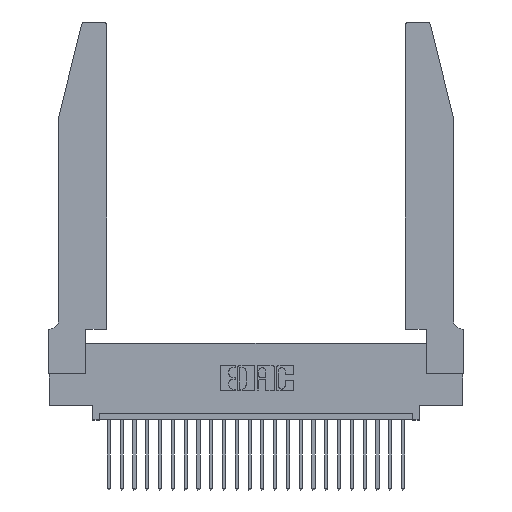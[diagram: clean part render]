
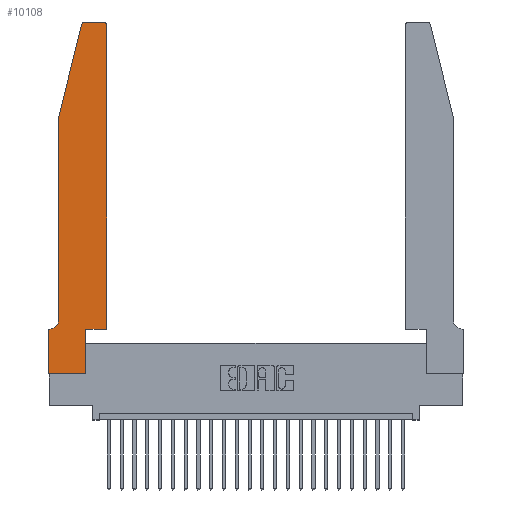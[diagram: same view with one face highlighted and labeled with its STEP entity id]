
A CAD part, top view. The second image highlights one B-rep face of the part: STEP entity #10108.
In plain terms, the highlighted planar face has unit normal (0, 0, 1).
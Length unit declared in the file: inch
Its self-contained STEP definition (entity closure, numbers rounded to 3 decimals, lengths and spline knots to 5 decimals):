
#411 = DIRECTION ( 'NONE',  ( 0., 0., 1. ) ) ;
#413 = LINE ( 'NONE', #1307, #14219 ) ;
#421 = CARTESIAN_POINT ( 'NONE',  ( 0.2605, 2.75, 0.37 ) ) ;
#437 = DIRECTION ( 'NONE',  ( 0., 1., 0. ) ) ;
#847 = VECTOR ( 'NONE', #10020, 39.37008 ) ;
#921 = EDGE_CURVE ( 'NONE', #11920, #24550, #14536, .T. ) ;
#956 = CARTESIAN_POINT ( 'NONE',  ( 0.4505, 0.35, 0.37 ) ) ;
#1104 = EDGE_CURVE ( 'NONE', #2616, #14932, #413, .T. ) ;
#1137 = VERTEX_POINT ( 'NONE', #4979 ) ;
#1307 = CARTESIAN_POINT ( 'NONE',  ( 0., 0., 0.37 ) ) ;
#1607 = EDGE_CURVE ( 'NONE', #24550, #12970, #20938, .T. ) ;
#1717 = CARTESIAN_POINT ( 'NONE',  ( 0.284, 2.75, 0.37 ) ) ;
#2001 = CIRCLE ( 'NONE', #3855, 0.07 ) ;
#2033 = DIRECTION ( 'NONE',  ( 0., 0., 1. ) ) ;
#2428 = CARTESIAN_POINT ( 'NONE',  ( 0.0755, 2., 0.37 ) ) ;
#2616 = VERTEX_POINT ( 'NONE', #12518 ) ;
#2748 = ORIENTED_EDGE ( 'NONE', *, *, #10962, .T. ) ;
#2857 = VECTOR ( 'NONE', #20580, 39.37008 ) ;
#3002 = FACE_OUTER_BOUND ( 'NONE', #3259, .T. ) ;
#3259 = EDGE_LOOP ( 'NONE', ( #16707, #22933, #7563, #19313, #4083, #14543, #13336, #22594, #2748, #11919, #10483, #11389 ) ) ;
#3855 = AXIS2_PLACEMENT_3D ( 'NONE', #16775, #8666, #4684 ) ;
#3896 = CIRCLE ( 'NONE', #11176, 0.03 ) ;
#3899 = CIRCLE ( 'NONE', #13970, 0.03 ) ;
#4083 = ORIENTED_EDGE ( 'NONE', *, *, #6516, .T. ) ;
#4098 = CARTESIAN_POINT ( 'NONE',  ( 0.4505, 0.35, 0.37 ) ) ;
#4505 = EDGE_CURVE ( 'NONE', #8027, #13186, #14383, .T. ) ;
#4684 = DIRECTION ( 'NONE',  ( -1., 0., 0. ) ) ;
#4979 = CARTESIAN_POINT ( 'NONE',  ( 0., 0.35, 0.37 ) ) ;
#5818 = CARTESIAN_POINT ( 'NONE',  ( 0.284, 2.72, 0.37 ) ) ;
#6023 = CARTESIAN_POINT ( 'NONE',  ( 0.0755, 0.42, 0.37 ) ) ;
#6516 = EDGE_CURVE ( 'NONE', #13186, #13162, #2001, .T. ) ;
#6771 = CARTESIAN_POINT ( 'NONE',  ( 0.4205, 2.75, 0.37 ) ) ;
#7563 = ORIENTED_EDGE ( 'NONE', *, *, #13368, .T. ) ;
#7775 = LINE ( 'NONE', #421, #24602 ) ;
#7932 = VECTOR ( 'NONE', #11212, 39.37008 ) ;
#8027 = VERTEX_POINT ( 'NONE', #2428 ) ;
#8551 = VECTOR ( 'NONE', #12024, 39.37008 ) ;
#8628 = CARTESIAN_POINT ( 'NONE',  ( 0.2865, 0.35, 0.37 ) ) ;
#8666 = DIRECTION ( 'NONE',  ( 0., 0., -1. ) ) ;
#9641 = VECTOR ( 'NONE', #20175, 39.37008 ) ;
#9778 = LINE ( 'NONE', #21817, #8551 ) ;
#10020 = DIRECTION ( 'NONE',  ( 0., -1., 0. ) ) ;
#10108 = ADVANCED_FACE ( 'NONE', ( #3002 ), #24135, .T. ) ;
#10483 = ORIENTED_EDGE ( 'NONE', *, *, #1607, .T. ) ;
#10665 = AXIS2_PLACEMENT_3D ( 'NONE', #18145, #411, #14136 ) ;
#10690 = CARTESIAN_POINT ( 'NONE',  ( 0.4205, 2.72, 0.37 ) ) ;
#10962 = EDGE_CURVE ( 'NONE', #14932, #11920, #9778, .T. ) ;
#11070 = EDGE_CURVE ( 'NONE', #13162, #1137, #13136, .T. ) ;
#11176 = AXIS2_PLACEMENT_3D ( 'NONE', #5818, #2033, #17178 ) ;
#11212 = DIRECTION ( 'NONE',  ( -1., 0., 0. ) ) ;
#11364 = EDGE_CURVE ( 'NONE', #12970, #16955, #3899, .T. ) ;
#11389 = ORIENTED_EDGE ( 'NONE', *, *, #11364, .T. ) ;
#11906 = VECTOR ( 'NONE', #22749, 39.37008 ) ;
#11919 = ORIENTED_EDGE ( 'NONE', *, *, #921, .T. ) ;
#11920 = VERTEX_POINT ( 'NONE', #8628 ) ;
#12024 = DIRECTION ( 'NONE',  ( 0., 1., 0. ) ) ;
#12040 = VECTOR ( 'NONE', #437, 39.37008 ) ;
#12518 = CARTESIAN_POINT ( 'NONE',  ( 0., 0., 0.37 ) ) ;
#12706 = CARTESIAN_POINT ( 'NONE',  ( 0.0755, 2., 0.37 ) ) ;
#12881 = CARTESIAN_POINT ( 'NONE',  ( 0.0755, 2., 0.37 ) ) ;
#12970 = VERTEX_POINT ( 'NONE', #19257 ) ;
#13136 = LINE ( 'NONE', #24634, #7932 ) ;
#13162 = VERTEX_POINT ( 'NONE', #17018 ) ;
#13186 = VERTEX_POINT ( 'NONE', #6023 ) ;
#13336 = ORIENTED_EDGE ( 'NONE', *, *, #16733, .T. ) ;
#13368 = EDGE_CURVE ( 'NONE', #25343, #8027, #20967, .T. ) ;
#13970 = AXIS2_PLACEMENT_3D ( 'NONE', #10690, #24046, #18549 ) ;
#14125 = CARTESIAN_POINT ( 'NONE',  ( 0., 0., 0.37 ) ) ;
#14136 = DIRECTION ( 'NONE',  ( 1., 0., 0. ) ) ;
#14219 = VECTOR ( 'NONE', #19035, 39.37008 ) ;
#14383 = LINE ( 'NONE', #12706, #11906 ) ;
#14536 = LINE ( 'NONE', #956, #2857 ) ;
#14543 = ORIENTED_EDGE ( 'NONE', *, *, #11070, .T. ) ;
#14932 = VERTEX_POINT ( 'NONE', #17309 ) ;
#15155 = VERTEX_POINT ( 'NONE', #1717 ) ;
#16651 = EDGE_CURVE ( 'NONE', #15155, #25343, #3896, .T. ) ;
#16707 = ORIENTED_EDGE ( 'NONE', *, *, #22264, .T. ) ;
#16733 = EDGE_CURVE ( 'NONE', #1137, #2616, #23229, .T. ) ;
#16775 = CARTESIAN_POINT ( 'NONE',  ( 0.0055, 0.42, 0.37 ) ) ;
#16955 = VERTEX_POINT ( 'NONE', #6771 ) ;
#17018 = CARTESIAN_POINT ( 'NONE',  ( 0.0055, 0.35, 0.37 ) ) ;
#17178 = DIRECTION ( 'NONE',  ( 1., 0., 0. ) ) ;
#17309 = CARTESIAN_POINT ( 'NONE',  ( 0.2865, 0., 0.37 ) ) ;
#18066 = DIRECTION ( 'NONE',  ( -1., 0., 0. ) ) ;
#18145 = CARTESIAN_POINT ( 'NONE',  ( 0., 0.35, 0.37 ) ) ;
#18549 = DIRECTION ( 'NONE',  ( 1., 0., 0. ) ) ;
#19035 = DIRECTION ( 'NONE',  ( 1., 0., 0. ) ) ;
#19216 = CARTESIAN_POINT ( 'NONE',  ( 0.25487, 2.72718, 0.37 ) ) ;
#19257 = CARTESIAN_POINT ( 'NONE',  ( 0.4505, 2.72, 0.37 ) ) ;
#19313 = ORIENTED_EDGE ( 'NONE', *, *, #4505, .T. ) ;
#20175 = DIRECTION ( 'NONE',  ( -0.239, -0.971, 0. ) ) ;
#20580 = DIRECTION ( 'NONE',  ( 1., 0., 0. ) ) ;
#20866 = CARTESIAN_POINT ( 'NONE',  ( 0.4505, 0.35, 0.37 ) ) ;
#20938 = LINE ( 'NONE', #4098, #12040 ) ;
#20967 = LINE ( 'NONE', #12881, #9641 ) ;
#21817 = CARTESIAN_POINT ( 'NONE',  ( 0.2865, 0.35, 0.37 ) ) ;
#22264 = EDGE_CURVE ( 'NONE', #16955, #15155, #7775, .T. ) ;
#22594 = ORIENTED_EDGE ( 'NONE', *, *, #1104, .T. ) ;
#22749 = DIRECTION ( 'NONE',  ( 0., -1., 0. ) ) ;
#22933 = ORIENTED_EDGE ( 'NONE', *, *, #16651, .T. ) ;
#23229 = LINE ( 'NONE', #14125, #847 ) ;
#24046 = DIRECTION ( 'NONE',  ( 0., 0., 1. ) ) ;
#24135 = PLANE ( 'NONE',  #10665 ) ;
#24550 = VERTEX_POINT ( 'NONE', #20866 ) ;
#24602 = VECTOR ( 'NONE', #18066, 39.37008 ) ;
#24634 = CARTESIAN_POINT ( 'NONE',  ( 0.0755, 0.35, 0.37 ) ) ;
#25343 = VERTEX_POINT ( 'NONE', #19216 ) ;
